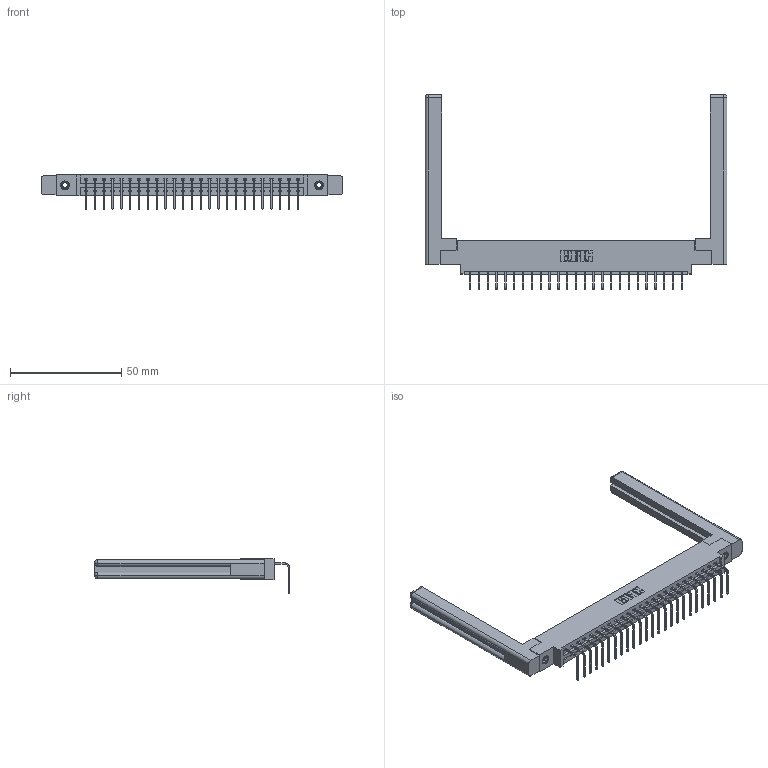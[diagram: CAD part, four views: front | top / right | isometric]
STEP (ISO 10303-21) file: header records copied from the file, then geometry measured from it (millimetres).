
FILE_DESCRIPTION (( 'STEP AP203' ), '1' );
FILE_NAME ('387-025-558-658.STEP', '2019-10-07T18:42:46', ( '' ), ( '' ), 'SwSTEP 2.0', 'SolidWorks 2016', '' );
FILE_SCHEMA (( 'CONFIG_CONTROL_DESIGN' ));
Length unit declared in the file: inch
Products named in the file (5): 307-220-058; 337 Part_0.170 Offset - 0.156 Dia-TI; 345-250-001_345-250-001-102; 345-292-001_558 Tail - 2; 387-025-558-658
Assembly tree (30 placements, depth 2):
  387-025-558-658
    337 Part_0.170 Offset - 0.156 Dia-TI
    345-292-001_558 Tail - 2  x25
    345-250-001_345-250-001-102  x2
    307-220-058  x2
Bounding box: 135.69 x 87.57 x 15.37 mm (x, y, z)
Volume: 21017.6 mm3; surface area: 20044.3 mm2
Topology: 30 solids, 30 shells, 1860 faces, 5527 edges, 3638 vertices
Faces by surface type: plane 1358, cylinder 478, cone 12, torus 12
Entity records: 23632 total; most frequent: CARTESIAN_POINT 4116, ORIENTED_EDGE 4016, DIRECTION 3518, EDGE_CURVE 2008, LINE 1832, VECTOR 1832, VERTEX_POINT 1330, AXIS2_PLACEMENT_3D 843
